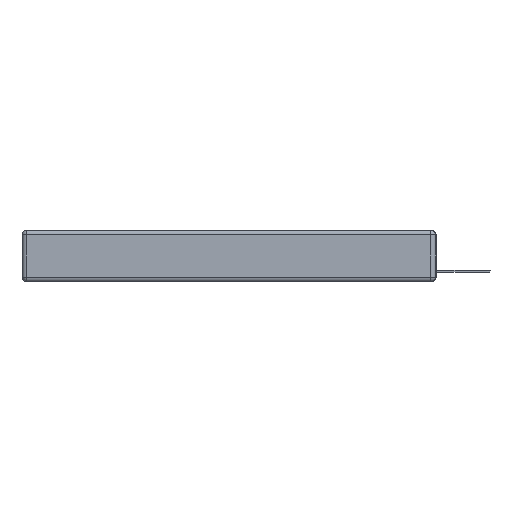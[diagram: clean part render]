
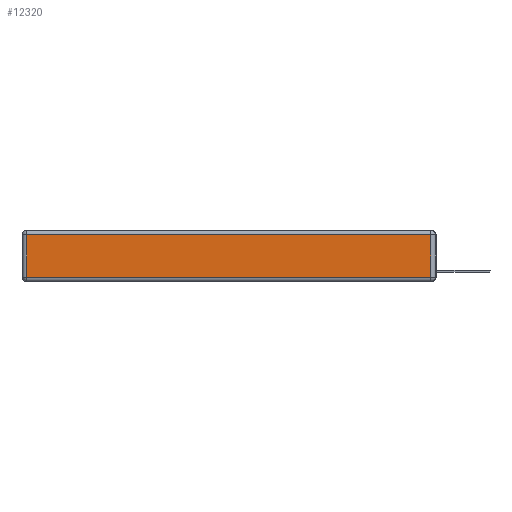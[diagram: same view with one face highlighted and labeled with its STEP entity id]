
A CAD part, left-side view. The second image highlights one B-rep face of the part: STEP entity #12320.
In plain terms, the highlighted planar face has unit normal (-1, 0, 0).
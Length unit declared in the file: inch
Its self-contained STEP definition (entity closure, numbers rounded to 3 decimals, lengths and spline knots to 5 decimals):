
#518 = CARTESIAN_POINT ( 'NONE',  ( 0., 0.03, -0.343 ) ) ;
#1962 = LINE ( 'NONE', #13911, #9806 ) ;
#3484 = LINE ( 'NONE', #13666, #7697 ) ;
#4107 = FACE_OUTER_BOUND ( 'NONE', #12097, .T. ) ;
#4246 = CARTESIAN_POINT ( 'NONE',  ( 0., 2.72, -0.03 ) ) ;
#4332 = PLANE ( 'NONE',  #12469 ) ;
#4575 = VERTEX_POINT ( 'NONE', #16952 ) ;
#5134 = VERTEX_POINT ( 'NONE', #7121 ) ;
#5387 = LINE ( 'NONE', #518, #17962 ) ;
#5410 = DIRECTION ( 'NONE',  ( 0., -1., 0. ) ) ;
#7121 = CARTESIAN_POINT ( 'NONE',  ( 0., 0.03, -0.313 ) ) ;
#7416 = EDGE_CURVE ( 'NONE', #19711, #5134, #1962, .T. ) ;
#7697 = VECTOR ( 'NONE', #12218, 39.37008 ) ;
#8453 = VECTOR ( 'NONE', #9257, 39.37008 ) ;
#9257 = DIRECTION ( 'NONE',  ( 0., 1., 0. ) ) ;
#9363 = CARTESIAN_POINT ( 'NONE',  ( 0., 2.75, -0.03 ) ) ;
#9613 = ORIENTED_EDGE ( 'NONE', *, *, #16332, .T. ) ;
#9806 = VECTOR ( 'NONE', #5410, 39.37008 ) ;
#11283 = CARTESIAN_POINT ( 'NONE',  ( 0., 2.72, -0.313 ) ) ;
#11870 = ORIENTED_EDGE ( 'NONE', *, *, #7416, .T. ) ;
#12097 = EDGE_LOOP ( 'NONE', ( #11870, #9613, #18392, #14310 ) ) ;
#12117 = DIRECTION ( 'NONE',  ( 0., 0., 1. ) ) ;
#12218 = DIRECTION ( 'NONE',  ( 0., 0., -1. ) ) ;
#12320 = ADVANCED_FACE ( 'NONE', ( #4107 ), #4332, .T. ) ;
#12469 = AXIS2_PLACEMENT_3D ( 'NONE', #16134, #12518, #21024 ) ;
#12518 = DIRECTION ( 'NONE',  ( -1., 0., 0. ) ) ;
#13666 = CARTESIAN_POINT ( 'NONE',  ( 0., 2.72, -0.343 ) ) ;
#13911 = CARTESIAN_POINT ( 'NONE',  ( 0., 0., -0.313 ) ) ;
#14310 = ORIENTED_EDGE ( 'NONE', *, *, #14805, .T. ) ;
#14805 = EDGE_CURVE ( 'NONE', #14908, #19711, #3484, .T. ) ;
#14908 = VERTEX_POINT ( 'NONE', #4246 ) ;
#16134 = CARTESIAN_POINT ( 'NONE',  ( 0., 0., -0.343 ) ) ;
#16332 = EDGE_CURVE ( 'NONE', #5134, #4575, #5387, .T. ) ;
#16952 = CARTESIAN_POINT ( 'NONE',  ( 0., 0.03, -0.03 ) ) ;
#17642 = LINE ( 'NONE', #9363, #8453 ) ;
#17776 = EDGE_CURVE ( 'NONE', #4575, #14908, #17642, .T. ) ;
#17962 = VECTOR ( 'NONE', #12117, 39.37008 ) ;
#18392 = ORIENTED_EDGE ( 'NONE', *, *, #17776, .T. ) ;
#19711 = VERTEX_POINT ( 'NONE', #11283 ) ;
#21024 = DIRECTION ( 'NONE',  ( 0., 0., 1. ) ) ;
